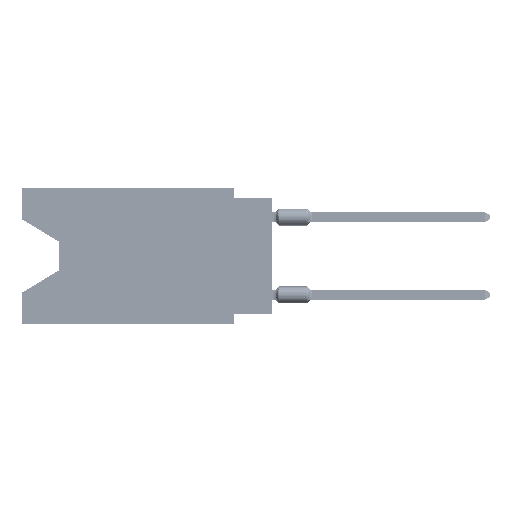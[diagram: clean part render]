
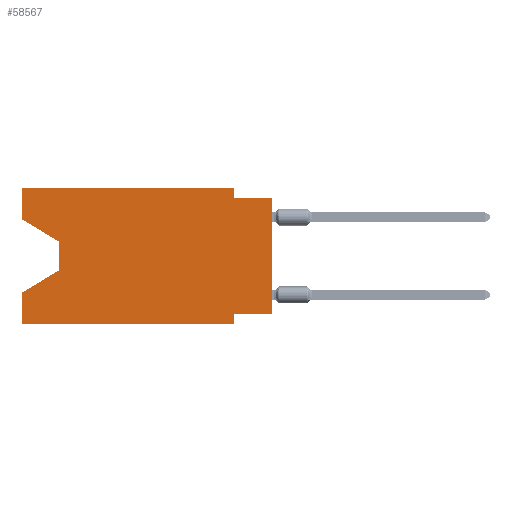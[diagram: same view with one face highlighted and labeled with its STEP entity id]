
A CAD part, left-side view. The second image highlights one B-rep face of the part: STEP entity #58567.
In plain terms, the highlighted planar face has unit normal (-1, 0, 0).
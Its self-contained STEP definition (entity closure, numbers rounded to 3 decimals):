
#618 = LINE ( 'NONE', #37149, #34016 ) ;
#1049 = ORIENTED_EDGE ( 'NONE', *, *, #11246, .F. ) ;
#1993 = EDGE_CURVE ( 'NONE', #53260, #61085, #618, .T. ) ;
#2511 = VERTEX_POINT ( 'NONE', #12444 ) ;
#2541 = DIRECTION ( 'NONE',  ( 0., 0., -1. ) ) ;
#2677 = LINE ( 'NONE', #75306, #63240 ) ;
#2967 = EDGE_CURVE ( 'NONE', #54097, #63086, #2677, .T. ) ;
#3262 = CARTESIAN_POINT ( 'NONE',  ( 0., 0., -0.635 ) ) ;
#3509 = VECTOR ( 'NONE', #12564, 1000. ) ;
#5497 = LINE ( 'NONE', #29725, #63069 ) ;
#5534 = LINE ( 'NONE', #52783, #69184 ) ;
#6440 = DIRECTION ( 'NONE',  ( 0., 0., -1. ) ) ;
#6982 = DIRECTION ( 'NONE',  ( 0., 0., 1. ) ) ;
#8673 = EDGE_CURVE ( 'NONE', #52952, #71143, #30593, .T. ) ;
#9181 = VECTOR ( 'NONE', #38107, 1000. ) ;
#9457 = ORIENTED_EDGE ( 'NONE', *, *, #68536, .F. ) ;
#10309 = CARTESIAN_POINT ( 'NONE',  ( 0., 0., -8.255 ) ) ;
#10544 = DIRECTION ( 'NONE',  ( 0., -1., 0. ) ) ;
#11246 = EDGE_CURVE ( 'NONE', #53260, #52952, #57555, .T. ) ;
#12444 = CARTESIAN_POINT ( 'NONE',  ( 0., 16.383, -2.038 ) ) ;
#12564 = DIRECTION ( 'NONE',  ( 0., -0.855, -0.519 ) ) ;
#12962 = DIRECTION ( 'NONE',  ( 0., 0., -1. ) ) ;
#13506 = VECTOR ( 'NONE', #44976, 1000. ) ;
#15103 = VECTOR ( 'NONE', #10544, 1000. ) ;
#15876 = DIRECTION ( 'NONE',  ( 0., 1., 0. ) ) ;
#16056 = EDGE_CURVE ( 'NONE', #45672, #63086, #5534, .T. ) ;
#16793 = ORIENTED_EDGE ( 'NONE', *, *, #1993, .T. ) ;
#17182 = EDGE_CURVE ( 'NONE', #26409, #43114, #73983, .T. ) ;
#17668 = CARTESIAN_POINT ( 'NONE',  ( 0., 2.54, -0.635 ) ) ;
#17817 = DIRECTION ( 'NONE',  ( 0., -1., 0. ) ) ;
#19388 = DIRECTION ( 'NONE',  ( 0., 0., 1. ) ) ;
#19865 = CARTESIAN_POINT ( 'NONE',  ( 0., 2.54, -8.89 ) ) ;
#20331 = EDGE_CURVE ( 'NONE', #2511, #41354, #47498, .T. ) ;
#20985 = VECTOR ( 'NONE', #12962, 1000. ) ;
#24018 = LINE ( 'NONE', #59741, #15103 ) ;
#24138 = EDGE_CURVE ( 'NONE', #41354, #45672, #43328, .T. ) ;
#25907 = CARTESIAN_POINT ( 'NONE',  ( 0., 13.97, -5.385 ) ) ;
#26409 = VERTEX_POINT ( 'NONE', #48122 ) ;
#27536 = PLANE ( 'NONE',  #36918 ) ;
#28100 = EDGE_CURVE ( 'NONE', #72980, #61085, #24018, .T. ) ;
#28331 = DIRECTION ( 'NONE',  ( 1., 0., 0. ) ) ;
#29534 = CARTESIAN_POINT ( 'NONE',  ( 0., 2.54, -8.89 ) ) ;
#29725 = CARTESIAN_POINT ( 'NONE',  ( 0., 16.383, -8.89 ) ) ;
#30593 = LINE ( 'NONE', #19865, #9181 ) ;
#33499 = CARTESIAN_POINT ( 'NONE',  ( 0., 16.383, 0. ) ) ;
#34016 = VECTOR ( 'NONE', #6982, 1000. ) ;
#36849 = LINE ( 'NONE', #55893, #37766 ) ;
#36918 = AXIS2_PLACEMENT_3D ( 'NONE', #33499, #28331, #2541 ) ;
#37149 = CARTESIAN_POINT ( 'NONE',  ( 0., 0., 0. ) ) ;
#37766 = VECTOR ( 'NONE', #19388, 1000. ) ;
#38107 = DIRECTION ( 'NONE',  ( 0., 0., -1. ) ) ;
#38695 = EDGE_CURVE ( 'NONE', #54097, #71143, #5497, .T. ) ;
#38772 = EDGE_CURVE ( 'NONE', #2511, #26409, #36849, .T. ) ;
#39833 = FACE_OUTER_BOUND ( 'NONE', #77458, .T. ) ;
#41354 = VERTEX_POINT ( 'NONE', #52719 ) ;
#41827 = ORIENTED_EDGE ( 'NONE', *, *, #38695, .T. ) ;
#42331 = CARTESIAN_POINT ( 'NONE',  ( 0., 16.383, -2.038 ) ) ;
#43114 = VERTEX_POINT ( 'NONE', #60546 ) ;
#43328 = LINE ( 'NONE', #65973, #75519 ) ;
#43500 = LINE ( 'NONE', #55416, #20985 ) ;
#44976 = DIRECTION ( 'NONE',  ( 0., -1., 0. ) ) ;
#45672 = VERTEX_POINT ( 'NONE', #25907 ) ;
#47191 = CARTESIAN_POINT ( 'NONE',  ( 0., 0., -8.255 ) ) ;
#47219 = DIRECTION ( 'NONE',  ( 0., 0.855, -0.519 ) ) ;
#47498 = LINE ( 'NONE', #42331, #3509 ) ;
#48066 = ORIENTED_EDGE ( 'NONE', *, *, #2967, .F. ) ;
#48122 = CARTESIAN_POINT ( 'NONE',  ( 0., 16.383, 0. ) ) ;
#52719 = CARTESIAN_POINT ( 'NONE',  ( 0., 13.97, -3.505 ) ) ;
#52783 = CARTESIAN_POINT ( 'NONE',  ( 0., 13.97, -5.385 ) ) ;
#52952 = VERTEX_POINT ( 'NONE', #54026 ) ;
#53260 = VERTEX_POINT ( 'NONE', #47191 ) ;
#54026 = CARTESIAN_POINT ( 'NONE',  ( 0., 2.54, -8.255 ) ) ;
#54097 = VERTEX_POINT ( 'NONE', #65655 ) ;
#55416 = CARTESIAN_POINT ( 'NONE',  ( 0., 2.54, 0. ) ) ;
#55893 = CARTESIAN_POINT ( 'NONE',  ( 0., 16.383, 0. ) ) ;
#56395 = ORIENTED_EDGE ( 'NONE', *, *, #16056, .T. ) ;
#56800 = ORIENTED_EDGE ( 'NONE', *, *, #20331, .T. ) ;
#57555 = LINE ( 'NONE', #10309, #59759 ) ;
#58567 = ADVANCED_FACE ( 'NONE', ( #39833 ), #27536, .F. ) ;
#59741 = CARTESIAN_POINT ( 'NONE',  ( 0., 0., -0.635 ) ) ;
#59759 = VECTOR ( 'NONE', #15876, 1000. ) ;
#60546 = CARTESIAN_POINT ( 'NONE',  ( 0., 2.54, 0. ) ) ;
#61085 = VERTEX_POINT ( 'NONE', #3262 ) ;
#63031 = ORIENTED_EDGE ( 'NONE', *, *, #24138, .T. ) ;
#63069 = VECTOR ( 'NONE', #17817, 1000. ) ;
#63086 = VERTEX_POINT ( 'NONE', #69754 ) ;
#63235 = CARTESIAN_POINT ( 'NONE',  ( 0., 16.383, 0. ) ) ;
#63240 = VECTOR ( 'NONE', #69344, 1000. ) ;
#65655 = CARTESIAN_POINT ( 'NONE',  ( 0., 16.383, -8.89 ) ) ;
#65973 = CARTESIAN_POINT ( 'NONE',  ( 0., 13.97, -3.505 ) ) ;
#67010 = ORIENTED_EDGE ( 'NONE', *, *, #28100, .F. ) ;
#68270 = ORIENTED_EDGE ( 'NONE', *, *, #38772, .F. ) ;
#68536 = EDGE_CURVE ( 'NONE', #43114, #72980, #43500, .T. ) ;
#69184 = VECTOR ( 'NONE', #47219, 1000. ) ;
#69344 = DIRECTION ( 'NONE',  ( 0., 0., 1. ) ) ;
#69754 = CARTESIAN_POINT ( 'NONE',  ( 0., 16.383, -6.852 ) ) ;
#71143 = VERTEX_POINT ( 'NONE', #29534 ) ;
#71862 = ORIENTED_EDGE ( 'NONE', *, *, #8673, .F. ) ;
#72980 = VERTEX_POINT ( 'NONE', #17668 ) ;
#73983 = LINE ( 'NONE', #63235, #13506 ) ;
#75306 = CARTESIAN_POINT ( 'NONE',  ( 0., 16.383, 0. ) ) ;
#75519 = VECTOR ( 'NONE', #6440, 1000. ) ;
#75594 = ORIENTED_EDGE ( 'NONE', *, *, #17182, .F. ) ;
#77458 = EDGE_LOOP ( 'NONE', ( #56800, #63031, #56395, #48066, #41827, #71862, #1049, #16793, #67010, #9457, #75594, #68270 ) ) ;
